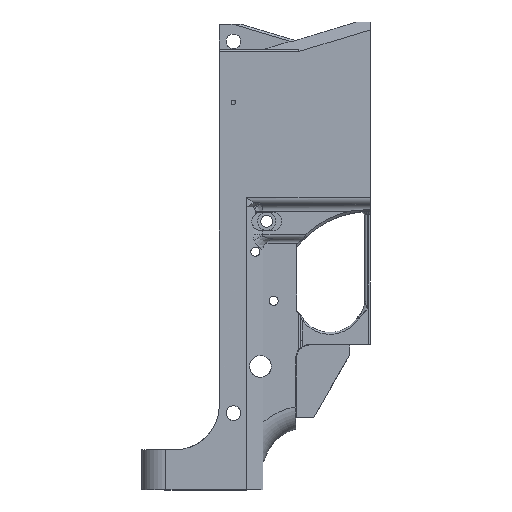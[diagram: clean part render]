
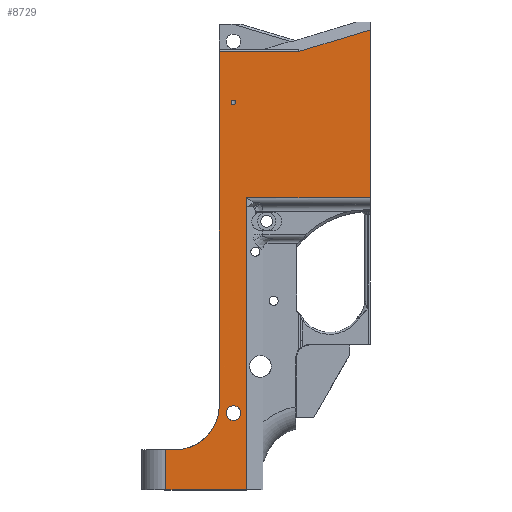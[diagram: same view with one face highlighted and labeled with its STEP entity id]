
A CAD part, left-side view. The second image highlights one B-rep face of the part: STEP entity #8729.
In plain terms, the highlighted planar face has unit normal (-1, 0, 0).
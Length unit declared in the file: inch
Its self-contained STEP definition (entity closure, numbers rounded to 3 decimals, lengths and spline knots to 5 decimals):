
#99=FACE_BOUND('',#1414,.T.);
#100=FACE_BOUND('',#1415,.T.);
#312=PLANE('',#9243);
#462=CIRCLE('',#9168,0.75984);
#493=CIRCLE('',#9244,0.039);
#494=CIRCLE('',#9245,0.039);
#495=CIRCLE('',#9246,0.125);
#927=FACE_OUTER_BOUND('',#1413,.T.);
#1413=EDGE_LOOP('',(#6585,#6586,#6587,#6588,#6589,#6590,#6591,#6592,#6593,
#6594,#6595,#6596));
#1414=EDGE_LOOP('',(#6597,#6598));
#1415=EDGE_LOOP('',(#6599));
#2047=B_SPLINE_CURVE_WITH_KNOTS('',3,(#21453,#21454,#21455,#21456,#21457,
#21458),.UNSPECIFIED.,.F.,.F.,(4,1,1,4),(0.,0.33333,0.66667,
1.),.UNSPECIFIED.);
#2313=LINE('',#21219,#2883);
#2349=LINE('',#21438,#2919);
#2350=LINE('',#21440,#2920);
#2351=LINE('',#21441,#2921);
#2352=LINE('',#21443,#2922);
#2353=LINE('',#21445,#2923);
#2354=LINE('',#21447,#2924);
#2355=LINE('',#21449,#2925);
#2356=LINE('',#21451,#2926);
#2357=LINE('',#21459,#2927);
#2883=VECTOR('',#10273,0.81541);
#2919=VECTOR('',#10339,1.28527);
#2920=VECTOR('',#10340,1.36014);
#2921=VECTOR('',#10341,6.06563);
#2922=VECTOR('',#10342,0.15611);
#2923=VECTOR('',#10343,0.3937);
#2924=VECTOR('',#10344,0.3937);
#2925=VECTOR('',#10345,1.69849);
#2926=VECTOR('',#10346,0.14801);
#2927=VECTOR('',#10347,2.12284);
#3594=VERTEX_POINT('',#20689);
#3595=VERTEX_POINT('',#20691);
#3666=VERTEX_POINT('',#21216);
#3667=VERTEX_POINT('',#21218);
#3707=VERTEX_POINT('',#21437);
#3708=VERTEX_POINT('',#21439);
#3709=VERTEX_POINT('',#21442);
#3710=VERTEX_POINT('',#21444);
#3711=VERTEX_POINT('',#21446);
#3712=VERTEX_POINT('',#21448);
#3713=VERTEX_POINT('',#21450);
#3714=VERTEX_POINT('',#21452);
#3715=VERTEX_POINT('',#21460);
#3716=VERTEX_POINT('',#21461);
#3717=VERTEX_POINT('',#21464);
#4609=EDGE_CURVE('',#3595,#3594,#462,.T.);
#4723=EDGE_CURVE('',#3667,#3666,#2313,.T.);
#4772=EDGE_CURVE('',#3666,#3707,#2349,.T.);
#4773=EDGE_CURVE('',#3708,#3707,#2350,.T.);
#4774=EDGE_CURVE('',#3595,#3708,#2351,.T.);
#4775=EDGE_CURVE('',#3709,#3594,#2352,.T.);
#4776=EDGE_CURVE('',#3709,#3710,#2353,.T.);
#4777=EDGE_CURVE('',#3710,#3711,#2354,.T.);
#4778=EDGE_CURVE('',#3712,#3711,#2355,.T.);
#4779=EDGE_CURVE('',#3712,#3713,#2356,.T.);
#4780=EDGE_CURVE('',#3713,#3714,#2047,.T.);
#4781=EDGE_CURVE('',#3714,#3667,#2357,.T.);
#4782=EDGE_CURVE('',#3715,#3716,#493,.T.);
#4783=EDGE_CURVE('',#3716,#3715,#494,.T.);
#4784=EDGE_CURVE('',#3717,#3717,#495,.T.);
#6585=ORIENTED_EDGE('',*,*,#4723,.T.);
#6586=ORIENTED_EDGE('',*,*,#4772,.T.);
#6587=ORIENTED_EDGE('',*,*,#4773,.F.);
#6588=ORIENTED_EDGE('',*,*,#4774,.F.);
#6589=ORIENTED_EDGE('',*,*,#4609,.T.);
#6590=ORIENTED_EDGE('',*,*,#4775,.F.);
#6591=ORIENTED_EDGE('',*,*,#4776,.T.);
#6592=ORIENTED_EDGE('',*,*,#4777,.T.);
#6593=ORIENTED_EDGE('',*,*,#4778,.F.);
#6594=ORIENTED_EDGE('',*,*,#4779,.T.);
#6595=ORIENTED_EDGE('',*,*,#4780,.T.);
#6596=ORIENTED_EDGE('',*,*,#4781,.T.);
#6597=ORIENTED_EDGE('',*,*,#4782,.T.);
#6598=ORIENTED_EDGE('',*,*,#4783,.T.);
#6599=ORIENTED_EDGE('',*,*,#4784,.T.);
#8729=ADVANCED_FACE('',(#927,#99,#100),#312,.T.);
#9168=AXIS2_PLACEMENT_3D('',#20692,#10073,#10074);
#9243=AXIS2_PLACEMENT_3D('',#21436,#10337,#10338);
#9244=AXIS2_PLACEMENT_3D('',#21462,#10348,#10349);
#9245=AXIS2_PLACEMENT_3D('',#21463,#10350,#10351);
#9246=AXIS2_PLACEMENT_3D('',#21465,#10352,#10353);
#10073=DIRECTION('center_axis',(1.,0.,0.));
#10074=DIRECTION('ref_axis',(0.,-1.,0.));
#10273=DIRECTION('',(0.,0.,1.));
#10337=DIRECTION('center_axis',(-1.,0.,0.));
#10338=DIRECTION('ref_axis',(0.,0.,1.));
#10339=DIRECTION('',(0.,0.957,-0.29));
#10340=DIRECTION('',(0.,-1.,0.));
#10341=DIRECTION('',(0.,0.,1.));
#10342=DIRECTION('',(0.,-1.,0.));
#10343=DIRECTION('',(0.,0.,-1.));
#10344=DIRECTION('',(0.,-1.,0.));
#10345=DIRECTION('',(0.,0.,-1.));
#10346=DIRECTION('',(0.,0.,1.));
#10347=DIRECTION('',(0.,-1.,0.));
#10348=DIRECTION('center_axis',(1.,0.,0.));
#10349=DIRECTION('ref_axis',(0.,1.,0.));
#10350=DIRECTION('center_axis',(1.,0.,0.));
#10351=DIRECTION('ref_axis',(0.,1.,0.));
#10352=DIRECTION('center_axis',(1.,0.,0.));
#10353=DIRECTION('ref_axis',(0.,0.,-1.));
#20689=CARTESIAN_POINT('',(-0.73097,2.09,-3.74484));
#20691=CARTESIAN_POINT('',(-0.73097,1.33016,-2.985));
#20692=CARTESIAN_POINT('Origin',(-0.73097,2.09,-2.985));
#21216=CARTESIAN_POINT('',(-0.73097,-1.26,3.45341));
#21218=CARTESIAN_POINT('',(-0.73097,-1.26,0.57169));
#21219=CARTESIAN_POINT('',(-0.73097,-1.26,2.63799));
#21436=CARTESIAN_POINT('Origin',(-0.73097,0.86284,2.41837));
#21437=CARTESIAN_POINT('',(-0.73097,-0.02998,3.08063));
#21438=CARTESIAN_POINT('',(-0.73097,-1.26,3.45341));
#21439=CARTESIAN_POINT('',(-0.73097,1.33016,3.08063));
#21440=CARTESIAN_POINT('',(-0.73097,1.33016,3.08063));
#21441=CARTESIAN_POINT('',(-0.73097,1.33016,-2.985));
#21442=CARTESIAN_POINT('',(-0.73097,2.24611,-3.74484));
#21443=CARTESIAN_POINT('',(-0.73097,2.24611,-3.74484));
#21444=CARTESIAN_POINT('',(-0.73097,2.24611,-4.43485));
#21445=CARTESIAN_POINT('',(-0.73097,2.24611,-4.238));
#21446=CARTESIAN_POINT('',(-0.73097,0.86284,-4.43485));
#21447=CARTESIAN_POINT('',(-0.73097,1.24392,-4.43485));
#21448=CARTESIAN_POINT('',(-0.73097,0.86284,0.4168));
#21449=CARTESIAN_POINT('',(-0.73097,0.86284,-2.50014));
#21450=CARTESIAN_POINT('',(-0.7309,0.86284,0.56481));
#21451=CARTESIAN_POINT('',(-0.73097,0.86284,0.4168));
#21452=CARTESIAN_POINT('',(-0.73097,0.86284,0.57169));
#21453=CARTESIAN_POINT('Ctrl Pts',(-0.7309,0.86284,
0.56481));
#21454=CARTESIAN_POINT('Ctrl Pts',(-0.7309,0.86284,
0.56557));
#21455=CARTESIAN_POINT('Ctrl Pts',(-0.731,0.86284,
0.5671));
#21456=CARTESIAN_POINT('Ctrl Pts',(-0.73096,0.86284,
0.56939));
#21457=CARTESIAN_POINT('Ctrl Pts',(-0.73097,0.86284,
0.57092));
#21458=CARTESIAN_POINT('Ctrl Pts',(-0.73097,0.86284,
0.57169));
#21459=CARTESIAN_POINT('',(-0.73097,0.86284,0.57169));
#21460=CARTESIAN_POINT('',(-0.73097,1.0505,2.21));
#21461=CARTESIAN_POINT('',(-0.73097,1.1285,2.21));
#21462=CARTESIAN_POINT('Origin',(-0.73097,1.0895,2.21));
#21463=CARTESIAN_POINT('Origin',(-0.73097,1.0895,2.21));
#21464=CARTESIAN_POINT('',(-0.73097,1.0895,-2.993));
#21465=CARTESIAN_POINT('Origin',(-0.73097,1.0895,-3.118));
